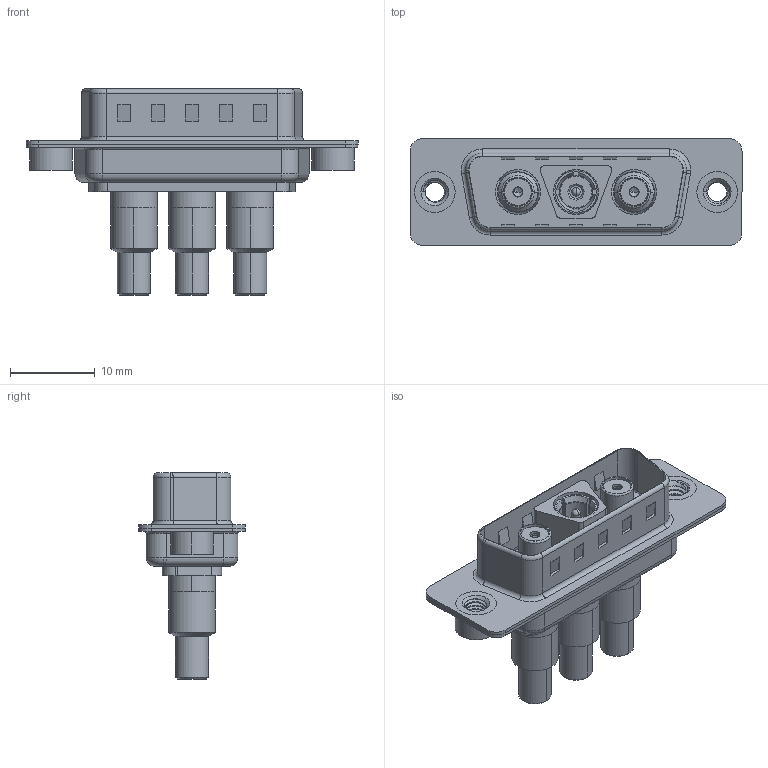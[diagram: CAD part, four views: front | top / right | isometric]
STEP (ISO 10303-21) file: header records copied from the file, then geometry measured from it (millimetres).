
FILE_DESCRIPTION (( 'STEP AP203' ), '1' );
FILE_NAME ('627-3WK3622-5NA.STEP', '2019-05-24T23:18:06', ( '' ), ( '' ), 'SwSTEP 2.0', 'SolidWorks 2016', '' );
FILE_SCHEMA (( 'CONFIG_CONTROL_DESIGN' ));
Length unit declared in the file: millimetre
Products named in the file (17): Co-Ax Plug Assy_SC; Co-Ax Jack_Solder Cup Tail; 627Combo Shell Front_15 Contacts; Insulator Socket; 627Combo Threaded Rivet_A; 627Combo Housing_3WK3; Insulator Socket 2; Solder Cover; Co-Ax Plug_Solder Cup Tail; 627Combo Shell Rear_15 Contacts; Socket_Solder Cup; Insulator Pin_Solder Cup Tail; Co-Ax Jack Assy_SC; Pin_Solder Cup; 627Combo Threaded Rivet_2; Locking Collar; 627-3WK3622-5NA
Assembly tree (19 placements, depth 3):
  627-3WK3622-5NA
    627Combo Housing_3WK3
    627Combo Shell Rear_15 Contacts
    627Combo Shell Front_15 Contacts
    627Combo Threaded Rivet_A
    Co-Ax Plug Assy_SC
      Co-Ax Plug_Solder Cup Tail
      Insulator Pin_Solder Cup Tail
      Pin_Solder Cup
      Locking Collar
      Solder Cover
    Co-Ax Jack Assy_SC  x2
      Co-Ax Jack_Solder Cup Tail
      Insulator Socket
      Insulator Socket 2
      Locking Collar
      Socket_Solder Cup
      Solder Cover
    627Combo Threaded Rivet_2
Bounding box: 39.15 x 12.6 x 24.3 mm (x, y, z)
Volume: 2343.8 mm3; surface area: 7393.5 mm2
Topology: 22 solids, 22 shells, 755 faces, 1804 edges, 1120 vertices
Faces by surface type: cylinder 329, plane 274, cone 76, torus 62, bspline 12, sphere 2
Entity records: 23012 total; most frequent: CARTESIAN_POINT 6612, DIRECTION 3206, ORIENTED_EDGE 2924, EDGE_CURVE 1462, AXIS2_PLACEMENT_3D 1234, VERTEX_POINT 920, VECTOR 738, LINE 738
